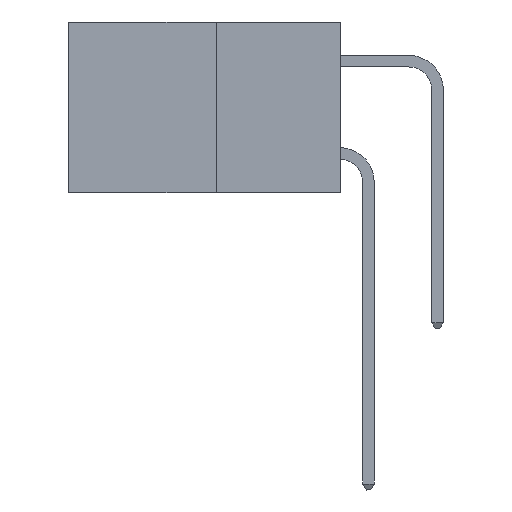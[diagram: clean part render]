
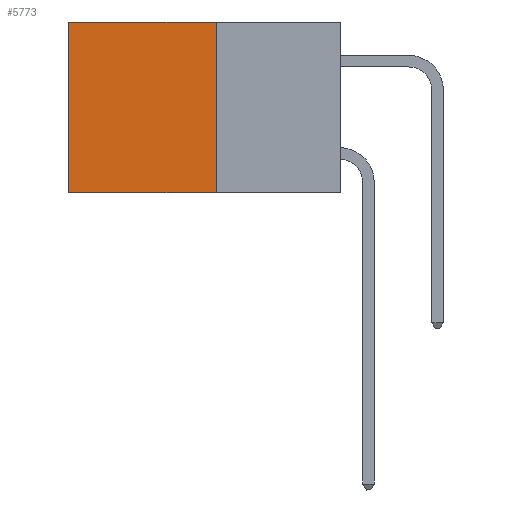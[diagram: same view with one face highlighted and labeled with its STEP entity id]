
A CAD part, left-side view. The second image highlights one B-rep face of the part: STEP entity #5773.
In plain terms, the highlighted planar face has unit normal (-1, 0, 0).
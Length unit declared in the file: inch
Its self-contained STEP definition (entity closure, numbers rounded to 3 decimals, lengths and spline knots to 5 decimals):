
#359 = ORIENTED_EDGE ( 'NONE', *, *, #2216, .T. ) ;
#422 = VECTOR ( 'NONE', #12028, 39.37008 ) ;
#1094 = VECTOR ( 'NONE', #3634, 39.37008 ) ;
#1212 = VECTOR ( 'NONE', #6758, 39.37008 ) ;
#1248 = EDGE_CURVE ( 'NONE', #2646, #9750, #10276, .T. ) ;
#1263 = CARTESIAN_POINT ( 'NONE',  ( 0.277, 0.27, -0.37 ) ) ;
#1842 = EDGE_CURVE ( 'NONE', #10919, #2033, #10638, .T. ) ;
#2033 = VERTEX_POINT ( 'NONE', #10896 ) ;
#2216 = EDGE_CURVE ( 'NONE', #2033, #9750, #4345, .T. ) ;
#2363 = CARTESIAN_POINT ( 'NONE',  ( 0.277, 0.59, -0.37 ) ) ;
#2423 = DIRECTION ( 'NONE',  ( 0., 0., -1. ) ) ;
#2646 = VERTEX_POINT ( 'NONE', #4709 ) ;
#2845 = CARTESIAN_POINT ( 'NONE',  ( 0.277, 0.27, -0.37 ) ) ;
#3244 = CARTESIAN_POINT ( 'NONE',  ( 0.277, 0.27, -0.37 ) ) ;
#3416 = EDGE_CURVE ( 'NONE', #10919, #2646, #8824, .T. ) ;
#3634 = DIRECTION ( 'NONE',  ( 0., 0., -1. ) ) ;
#4345 = LINE ( 'NONE', #2363, #1094 ) ;
#4709 = CARTESIAN_POINT ( 'NONE',  ( 0.277, 0.27, -0.37 ) ) ;
#4743 = EDGE_LOOP ( 'NONE', ( #359, #9607, #10502, #9673 ) ) ;
#4966 = FACE_OUTER_BOUND ( 'NONE', #4743, .T. ) ;
#5773 = ADVANCED_FACE ( 'NONE', ( #4966 ), #7105, .F. ) ;
#5803 = VECTOR ( 'NONE', #9895, 39.37008 ) ;
#6758 = DIRECTION ( 'NONE',  ( 0., 0., -1. ) ) ;
#7105 = PLANE ( 'NONE',  #9013 ) ;
#7861 = CARTESIAN_POINT ( 'NONE',  ( 0.277, 0.27, 0. ) ) ;
#8043 = DIRECTION ( 'NONE',  ( 1., 0., 0. ) ) ;
#8824 = LINE ( 'NONE', #2845, #1212 ) ;
#9013 = AXIS2_PLACEMENT_3D ( 'NONE', #1263, #8043, #2423 ) ;
#9030 = CARTESIAN_POINT ( 'NONE',  ( 0.277, 0.27, 0. ) ) ;
#9443 = CARTESIAN_POINT ( 'NONE',  ( 0.277, 0.59, -0.37 ) ) ;
#9607 = ORIENTED_EDGE ( 'NONE', *, *, #1248, .F. ) ;
#9673 = ORIENTED_EDGE ( 'NONE', *, *, #1842, .T. ) ;
#9750 = VERTEX_POINT ( 'NONE', #9443 ) ;
#9895 = DIRECTION ( 'NONE',  ( 0., 1., 0. ) ) ;
#10276 = LINE ( 'NONE', #3244, #422 ) ;
#10502 = ORIENTED_EDGE ( 'NONE', *, *, #3416, .F. ) ;
#10638 = LINE ( 'NONE', #9030, #5803 ) ;
#10896 = CARTESIAN_POINT ( 'NONE',  ( 0.277, 0.59, 0. ) ) ;
#10919 = VERTEX_POINT ( 'NONE', #7861 ) ;
#12028 = DIRECTION ( 'NONE',  ( 0., 1., 0. ) ) ;
